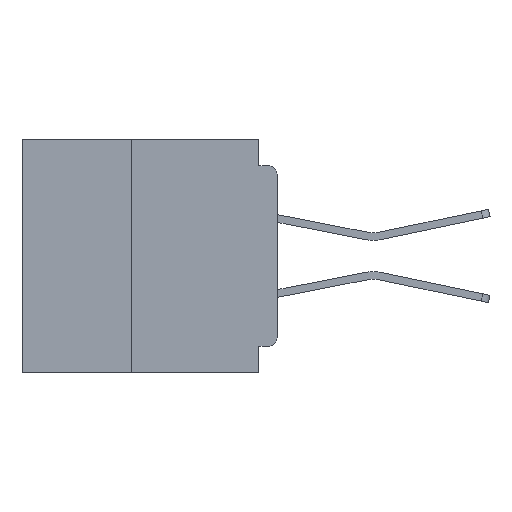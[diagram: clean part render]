
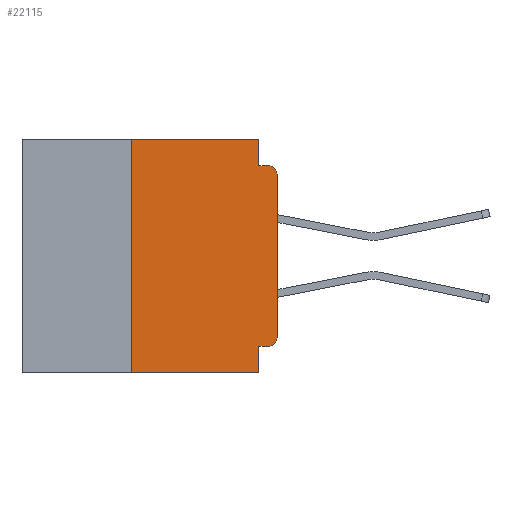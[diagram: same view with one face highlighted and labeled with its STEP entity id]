
A CAD part, left-side view. The second image highlights one B-rep face of the part: STEP entity #22115.
In plain terms, the highlighted planar face has unit normal (-1, 0, 0).
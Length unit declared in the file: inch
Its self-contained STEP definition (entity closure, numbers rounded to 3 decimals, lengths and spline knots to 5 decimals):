
#65 = ORIENTED_EDGE ( 'NONE', *, *, #53745, .F. ) ;
#867 = LINE ( 'NONE', #43363, #23963 ) ;
#1116 = CARTESIAN_POINT ( 'NONE',  ( 0., 0.031, 0. ) ) ;
#2649 = VERTEX_POINT ( 'NONE', #62316 ) ;
#2703 = EDGE_CURVE ( 'NONE', #40426, #58954, #57283, .T. ) ;
#3736 = VERTEX_POINT ( 'NONE', #54747 ) ;
#4568 = CARTESIAN_POINT ( 'NONE',  ( 0., 0.015, -0.045 ) ) ;
#4651 = CARTESIAN_POINT ( 'NONE',  ( 0., 0., -0.045 ) ) ;
#6435 = VECTOR ( 'NONE', #46690, 39.37008 ) ;
#7055 = CARTESIAN_POINT ( 'NONE',  ( 0., 0.437, 0. ) ) ;
#7712 = CARTESIAN_POINT ( 'NONE',  ( 0., 0.437, 0. ) ) ;
#7899 = DIRECTION ( 'NONE',  ( -1., 0., 0. ) ) ;
#9919 = LINE ( 'NONE', #39243, #19929 ) ;
#10748 = EDGE_CURVE ( 'NONE', #33741, #2649, #867, .T. ) ;
#11016 = CARTESIAN_POINT ( 'NONE',  ( 0., 0.031, 0. ) ) ;
#11699 = ORIENTED_EDGE ( 'NONE', *, *, #2703, .F. ) ;
#12034 = DIRECTION ( 'NONE',  ( 1., 0., 0. ) ) ;
#18478 = ORIENTED_EDGE ( 'NONE', *, *, #10748, .F. ) ;
#18741 = VECTOR ( 'NONE', #62731, 39.37008 ) ;
#19101 = CARTESIAN_POINT ( 'NONE',  ( 0., 0.031, -0.045 ) ) ;
#19460 = DIRECTION ( 'NONE',  ( -1., 0., 0. ) ) ;
#19929 = VECTOR ( 'NONE', #53721, 39.37008 ) ;
#21113 = VECTOR ( 'NONE', #57670, 39.37008 ) ;
#22115 = ADVANCED_FACE ( 'NONE', ( #57722 ), #36373, .F. ) ;
#22658 = VERTEX_POINT ( 'NONE', #45188 ) ;
#22664 = LINE ( 'NONE', #1116, #59598 ) ;
#23092 = CIRCLE ( 'NONE', #40122, 0.015 ) ;
#23121 = AXIS2_PLACEMENT_3D ( 'NONE', #48502, #19460, #53283 ) ;
#23299 = VERTEX_POINT ( 'NONE', #11016 ) ;
#23405 = VERTEX_POINT ( 'NONE', #55502 ) ;
#23962 = CARTESIAN_POINT ( 'NONE',  ( 0., 0.437, -0.4 ) ) ;
#23963 = VECTOR ( 'NONE', #57741, 39.37008 ) ;
#24346 = CARTESIAN_POINT ( 'NONE',  ( 0., 0.25, -0.4 ) ) ;
#24790 = EDGE_CURVE ( 'NONE', #23405, #23299, #53560, .T. ) ;
#25010 = ORIENTED_EDGE ( 'NONE', *, *, #49889, .T. ) ;
#25169 = LINE ( 'NONE', #34575, #49336 ) ;
#28046 = DIRECTION ( 'NONE',  ( 0., 0., -1. ) ) ;
#33189 = LINE ( 'NONE', #56876, #34743 ) ;
#33741 = VERTEX_POINT ( 'NONE', #43343 ) ;
#34025 = LINE ( 'NONE', #23962, #21113 ) ;
#34039 = EDGE_LOOP ( 'NONE', ( #35166, #62345, #11699, #34670, #47525, #65, #25010, #54512, #18478, #50781 ) ) ;
#34575 = CARTESIAN_POINT ( 'NONE',  ( 0., 0., 0. ) ) ;
#34638 = EDGE_CURVE ( 'NONE', #23299, #40426, #22664, .T. ) ;
#34670 = ORIENTED_EDGE ( 'NONE', *, *, #34638, .F. ) ;
#34743 = VECTOR ( 'NONE', #28046, 39.37008 ) ;
#35166 = ORIENTED_EDGE ( 'NONE', *, *, #48299, .T. ) ;
#36020 = EDGE_CURVE ( 'NONE', #2649, #47527, #33189, .T. ) ;
#36373 = PLANE ( 'NONE',  #47394 ) ;
#37206 = CARTESIAN_POINT ( 'NONE',  ( 0., 0.015, -0.06 ) ) ;
#38025 = EDGE_CURVE ( 'NONE', #33741, #22658, #59251, .T. ) ;
#39243 = CARTESIAN_POINT ( 'NONE',  ( 0., 0.25, -0.4 ) ) ;
#40046 = DIRECTION ( 'NONE',  ( 0., 0., -1. ) ) ;
#40122 = AXIS2_PLACEMENT_3D ( 'NONE', #37206, #7899, #42055 ) ;
#40426 = VERTEX_POINT ( 'NONE', #19101 ) ;
#42055 = DIRECTION ( 'NONE',  ( 0., 0., -1. ) ) ;
#43343 = CARTESIAN_POINT ( 'NONE',  ( 0., 0.015, -0.355 ) ) ;
#43363 = CARTESIAN_POINT ( 'NONE',  ( 0., 0., -0.355 ) ) ;
#45188 = CARTESIAN_POINT ( 'NONE',  ( 0., 0., -0.34 ) ) ;
#46074 = DIRECTION ( 'NONE',  ( 0., 0., -1. ) ) ;
#46690 = DIRECTION ( 'NONE',  ( 0., -1., 0. ) ) ;
#46963 = VERTEX_POINT ( 'NONE', #24346 ) ;
#47394 = AXIS2_PLACEMENT_3D ( 'NONE', #7055, #12034, #46074 ) ;
#47525 = ORIENTED_EDGE ( 'NONE', *, *, #24790, .F. ) ;
#47527 = VERTEX_POINT ( 'NONE', #48338 ) ;
#48299 = EDGE_CURVE ( 'NONE', #22658, #3736, #25169, .T. ) ;
#48338 = CARTESIAN_POINT ( 'NONE',  ( 0., 0.031, -0.4 ) ) ;
#48502 = CARTESIAN_POINT ( 'NONE',  ( 0., 0.015, -0.34 ) ) ;
#49336 = VECTOR ( 'NONE', #58486, 39.37008 ) ;
#49889 = EDGE_CURVE ( 'NONE', #46963, #47527, #34025, .T. ) ;
#50781 = ORIENTED_EDGE ( 'NONE', *, *, #38025, .T. ) ;
#52920 = EDGE_CURVE ( 'NONE', #3736, #58954, #23092, .T. ) ;
#53283 = DIRECTION ( 'NONE',  ( 0., 0., -1. ) ) ;
#53560 = LINE ( 'NONE', #7712, #6435 ) ;
#53721 = DIRECTION ( 'NONE',  ( 0., 0., 1. ) ) ;
#53745 = EDGE_CURVE ( 'NONE', #46963, #23405, #9919, .T. ) ;
#54512 = ORIENTED_EDGE ( 'NONE', *, *, #36020, .F. ) ;
#54747 = CARTESIAN_POINT ( 'NONE',  ( 0., 0., -0.06 ) ) ;
#55502 = CARTESIAN_POINT ( 'NONE',  ( 0., 0.25, 0. ) ) ;
#56876 = CARTESIAN_POINT ( 'NONE',  ( 0., 0.031, -0.4 ) ) ;
#57283 = LINE ( 'NONE', #4651, #18741 ) ;
#57670 = DIRECTION ( 'NONE',  ( 0., -1., 0. ) ) ;
#57722 = FACE_OUTER_BOUND ( 'NONE', #34039, .T. ) ;
#57741 = DIRECTION ( 'NONE',  ( 0., 1., 0. ) ) ;
#58486 = DIRECTION ( 'NONE',  ( 0., 0., 1. ) ) ;
#58954 = VERTEX_POINT ( 'NONE', #4568 ) ;
#59251 = CIRCLE ( 'NONE', #23121, 0.015 ) ;
#59598 = VECTOR ( 'NONE', #40046, 39.37008 ) ;
#62316 = CARTESIAN_POINT ( 'NONE',  ( 0., 0.031, -0.355 ) ) ;
#62345 = ORIENTED_EDGE ( 'NONE', *, *, #52920, .T. ) ;
#62731 = DIRECTION ( 'NONE',  ( 0., -1., 0. ) ) ;
